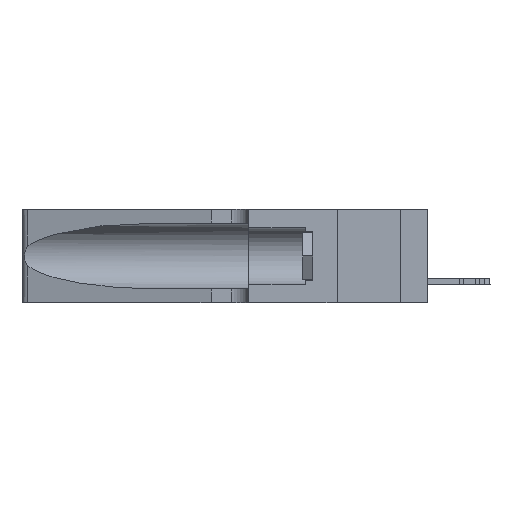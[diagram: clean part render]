
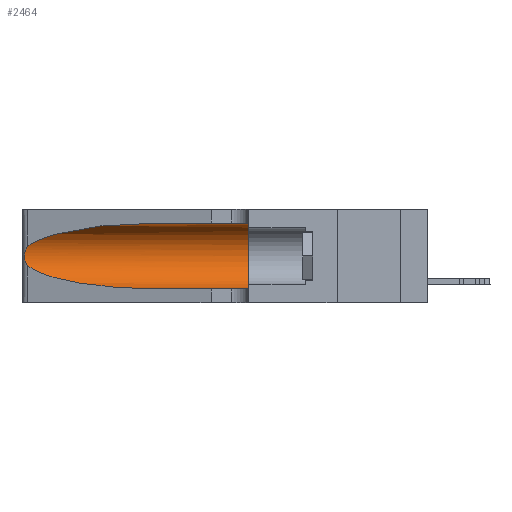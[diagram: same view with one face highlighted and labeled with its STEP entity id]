
A CAD part, left-side view. The second image highlights one B-rep face of the part: STEP entity #2464.
In plain terms, the highlighted cylindrical face has radius 3.308 mm (diameter 6.617 mm), a partial arc.
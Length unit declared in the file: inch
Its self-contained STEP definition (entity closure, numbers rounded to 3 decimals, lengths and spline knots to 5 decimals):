
#378 = VERTEX_POINT ( 'NONE', #13594 ) ;
#1025 = VERTEX_POINT ( 'NONE', #22100 ) ;
#1226 = CARTESIAN_POINT ( 'NONE',  ( 0.25787, 1.23484, 0.2124 ) ) ;
#1240 = AXIS2_PLACEMENT_3D ( 'NONE', #35807, #35470, #13379 ) ;
#1905 = CARTESIAN_POINT ( 'NONE',  ( 0.26017, 1.23833, 0.17102 ) ) ;
#2061 = EDGE_CURVE ( 'NONE', #15031, #30541, #33306, .T. ) ;
#2464 = ADVANCED_FACE ( 'NONE', ( #33833 ), #37876, .F. ) ;
#2756 = VERTEX_POINT ( 'NONE', #38422 ) ;
#2871 = ORIENTED_EDGE ( 'NONE', *, *, #2061, .T. ) ;
#3223 = ORIENTED_EDGE ( 'NONE', *, *, #6303, .F. ) ;
#4715 = DIRECTION ( 'NONE',  ( 0., 0., 1. ) ) ;
#5449 =( BOUNDED_CURVE ( )  B_SPLINE_CURVE ( 3, ( #28416, #32786, #33213, #11554 ),
 .UNSPECIFIED., .F., .T. ) 
 B_SPLINE_CURVE_WITH_KNOTS ( ( 4, 4 ),
 ( 3.44316, 4.71239 ),
 .UNSPECIFIED. ) 
 CURVE ( )  GEOMETRIC_REPRESENTATION_ITEM ( )  RATIONAL_B_SPLINE_CURVE ( ( 1., 0.87, 0.87, 1. ) ) 
 REPRESENTATION_ITEM ( '' )  );
#5955 = CIRCLE ( 'NONE', #8174, 0.13025 ) ;
#6303 = EDGE_CURVE ( 'NONE', #378, #30541, #5955, .T. ) ;
#7535 = CARTESIAN_POINT ( 'NONE',  ( 0.1305, 0.35, 0.05475 ) ) ;
#8174 = AXIS2_PLACEMENT_3D ( 'NONE', #33555, #29966, #4715 ) ;
#8628 = EDGE_LOOP ( 'NONE', ( #16229, #20983, #44974, #2871, #3223, #32276 ) ) ;
#11040 = CARTESIAN_POINT ( 'NONE',  ( 0.1305, 1.61858, 0.05475 ) ) ;
#11553 = VECTOR ( 'NONE', #25534, 39.37008 ) ;
#11554 = CARTESIAN_POINT ( 'NONE',  ( 0.1305, 0.72297, 0.05475 ) ) ;
#12518 = CARTESIAN_POINT ( 'NONE',  ( 0.25555, 1.22994, 0.2215 ) ) ;
#12945 = VERTEX_POINT ( 'NONE', #27154 ) ;
#13379 = DIRECTION ( 'NONE',  ( 0., 0., -1. ) ) ;
#13594 = CARTESIAN_POINT ( 'NONE',  ( 0.1305, 0.35, 0.31525 ) ) ;
#14742 = CARTESIAN_POINT ( 'NONE',  ( 0.2373, 1.15595, 0.28018 ) ) ;
#15031 = VERTEX_POINT ( 'NONE', #28133 ) ;
#16229 = ORIENTED_EDGE ( 'NONE', *, *, #22314, .T. ) ;
#17699 = CARTESIAN_POINT ( 'NONE',  ( 0.25555, 1.22993, 0.14849 ) ) ;
#18268 = CARTESIAN_POINT ( 'NONE',  ( 0.1305, 0.72297, 0.31525 ) ) ;
#20432 = B_SPLINE_CURVE_WITH_KNOTS ( 'NONE', 3,
 ( #22868, #12518, #38166, #1226, #26531, #35133, #27360, #42167, #1905, #38840, #39348, #43140, #17699, #46951 ),
 .UNSPECIFIED., .F., .F.,
 ( 4, 2, 2, 2, 2, 2, 4 ),
 ( 0., 0.00027, 0.00053, 0.00107, 0.0016, 0.00187, 0.00214 ),
 .UNSPECIFIED. ) ;
#20983 = ORIENTED_EDGE ( 'NONE', *, *, #28881, .T. ) ;
#21320 = DIRECTION ( 'NONE',  ( 0., -1., 0. ) ) ;
#22100 = CARTESIAN_POINT ( 'NONE',  ( 0.1305, 0.72297, 0.31525 ) ) ;
#22314 = EDGE_CURVE ( 'NONE', #1025, #2756, #39584, .T. ) ;
#22478 = CARTESIAN_POINT ( 'NONE',  ( 0.1305, 1.61858, 0.31525 ) ) ;
#22760 = CARTESIAN_POINT ( 'NONE',  ( 0.25487, 1.22718, 0.22369 ) ) ;
#22868 = CARTESIAN_POINT ( 'NONE',  ( 0.25487, 1.22718, 0.22369 ) ) ;
#25534 = DIRECTION ( 'NONE',  ( 0., -1., 0. ) ) ;
#26531 = CARTESIAN_POINT ( 'NONE',  ( 0.25854, 1.2359, 0.20912 ) ) ;
#26612 = EDGE_CURVE ( 'NONE', #1025, #378, #37361, .T. ) ;
#27154 = CARTESIAN_POINT ( 'NONE',  ( 0.25487, 1.22718, 0.14631 ) ) ;
#27360 = CARTESIAN_POINT ( 'NONE',  ( 0.26075, 1.23896, 0.19203 ) ) ;
#28133 = CARTESIAN_POINT ( 'NONE',  ( 0.1305, 0.72297, 0.05475 ) ) ;
#28416 = CARTESIAN_POINT ( 'NONE',  ( 0.25487, 1.22718, 0.14631 ) ) ;
#28881 = EDGE_CURVE ( 'NONE', #2756, #12945, #20432, .T. ) ;
#28935 = CARTESIAN_POINT ( 'NONE',  ( 0.18966, 0.96281, 0.31525 ) ) ;
#29966 = DIRECTION ( 'NONE',  ( 0., 1., 0. ) ) ;
#30541 = VERTEX_POINT ( 'NONE', #7535 ) ;
#32276 = ORIENTED_EDGE ( 'NONE', *, *, #26612, .F. ) ;
#32786 = CARTESIAN_POINT ( 'NONE',  ( 0.2373, 1.15595, 0.08982 ) ) ;
#33011 = EDGE_CURVE ( 'NONE', #12945, #15031, #5449, .T. ) ;
#33213 = CARTESIAN_POINT ( 'NONE',  ( 0.18966, 0.96281, 0.05475 ) ) ;
#33306 = LINE ( 'NONE', #11040, #43721 ) ;
#33555 = CARTESIAN_POINT ( 'NONE',  ( 0.1305, 0.35, 0.185 ) ) ;
#33833 = FACE_OUTER_BOUND ( 'NONE', #8628, .T. ) ;
#35133 = CARTESIAN_POINT ( 'NONE',  ( 0.26018, 1.23835, 0.19895 ) ) ;
#35470 = DIRECTION ( 'NONE',  ( 0., -1., 0. ) ) ;
#35807 = CARTESIAN_POINT ( 'NONE',  ( 0.1305, 1.61858, 0.185 ) ) ;
#37361 = LINE ( 'NONE', #22478, #11553 ) ;
#37876 = CYLINDRICAL_SURFACE ( 'NONE', #1240, 0.13025 ) ;
#38166 = CARTESIAN_POINT ( 'NONE',  ( 0.25639, 1.23184, 0.21858 ) ) ;
#38422 = CARTESIAN_POINT ( 'NONE',  ( 0.25487, 1.22718, 0.22369 ) ) ;
#38840 = CARTESIAN_POINT ( 'NONE',  ( 0.25856, 1.23593, 0.16098 ) ) ;
#39348 = CARTESIAN_POINT ( 'NONE',  ( 0.25789, 1.23486, 0.15765 ) ) ;
#39584 =( BOUNDED_CURVE ( )  B_SPLINE_CURVE ( 3, ( #18268, #28935, #14742, #22760 ),
 .UNSPECIFIED., .F., .T. ) 
 B_SPLINE_CURVE_WITH_KNOTS ( ( 4, 4 ),
 ( 1.5708, 2.84003 ),
 .UNSPECIFIED. ) 
 CURVE ( )  GEOMETRIC_REPRESENTATION_ITEM ( )  RATIONAL_B_SPLINE_CURVE ( ( 1., 0.87, 0.87, 1. ) ) 
 REPRESENTATION_ITEM ( '' )  );
#42167 = CARTESIAN_POINT ( 'NONE',  ( 0.26075, 1.23896, 0.178 ) ) ;
#43140 = CARTESIAN_POINT ( 'NONE',  ( 0.25639, 1.23186, 0.15144 ) ) ;
#43721 = VECTOR ( 'NONE', #21320, 39.37008 ) ;
#44974 = ORIENTED_EDGE ( 'NONE', *, *, #33011, .T. ) ;
#46951 = CARTESIAN_POINT ( 'NONE',  ( 0.25487, 1.22718, 0.14631 ) ) ;
